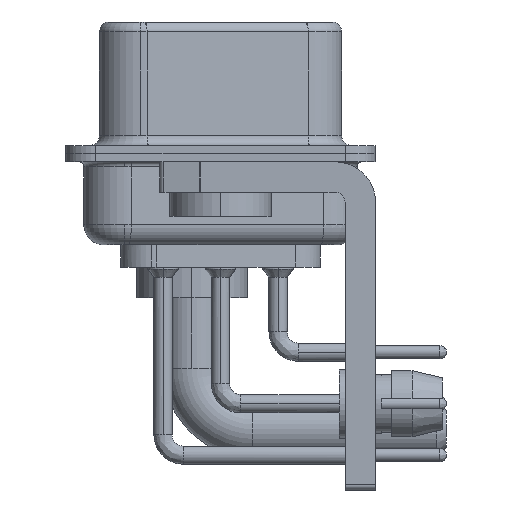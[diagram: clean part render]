
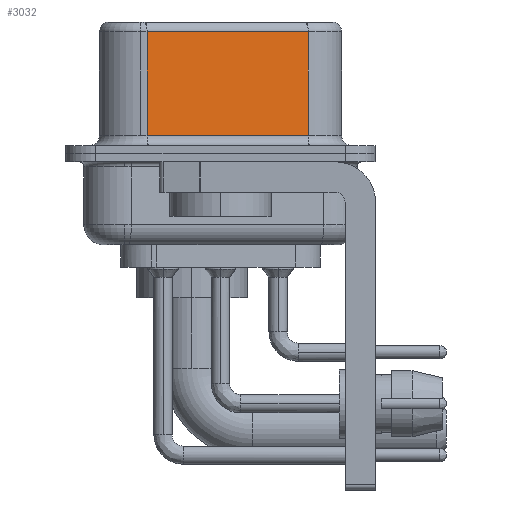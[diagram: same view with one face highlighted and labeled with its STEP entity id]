
A CAD part, left-side view. The second image highlights one B-rep face of the part: STEP entity #3032.
In plain terms, the highlighted planar face has unit normal (-0.985, -0.174, 0).
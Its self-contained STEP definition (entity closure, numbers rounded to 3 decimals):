
#808 = EDGE_CURVE ( 'NONE', #6352, #6250, #20248, .T. ) ;
#848 = VERTEX_POINT ( 'NONE', #11236 ) ;
#2903 = CARTESIAN_POINT ( 'NONE',  ( 5.132, -4.322, 6.02 ) ) ;
#3032 = ADVANCED_FACE ( 'NONE', ( #37084 ), #4297, .F. ) ;
#3439 = VECTOR ( 'NONE', #11633, 1000. ) ;
#4297 = PLANE ( 'NONE',  #15910 ) ;
#6250 = VERTEX_POINT ( 'NONE', #26858 ) ;
#6352 = VERTEX_POINT ( 'NONE', #2903 ) ;
#7738 = ORIENTED_EDGE ( 'NONE', *, *, #22018, .T. ) ;
#8629 = LINE ( 'NONE', #17471, #17528 ) ;
#11236 = CARTESIAN_POINT ( 'NONE',  ( 3.73, 3.628, 0.9 ) ) ;
#11633 = DIRECTION ( 'NONE',  ( -0.174, 0.985, 0. ) ) ;
#12528 = LINE ( 'NONE', #19176, #27349 ) ;
#12939 = DIRECTION ( 'NONE',  ( -0.174, 0.985, 0. ) ) ;
#13773 = EDGE_LOOP ( 'NONE', ( #18597, #20297, #7738, #29267 ) ) ;
#15324 = VERTEX_POINT ( 'NONE', #26922 ) ;
#15433 = VECTOR ( 'NONE', #23337, 1000. ) ;
#15910 = AXIS2_PLACEMENT_3D ( 'NONE', #18819, #22155, #12939 ) ;
#17471 = CARTESIAN_POINT ( 'NONE',  ( 5.132, -4.322, 0.9 ) ) ;
#17528 = VECTOR ( 'NONE', #32004, 1000. ) ;
#18180 = EDGE_CURVE ( 'NONE', #848, #15324, #8629, .T. ) ;
#18597 = ORIENTED_EDGE ( 'NONE', *, *, #21776, .F. ) ;
#18819 = CARTESIAN_POINT ( 'NONE',  ( 5.132, -4.322, 6.52 ) ) ;
#19176 = CARTESIAN_POINT ( 'NONE',  ( 3.73, 3.628, 6.52 ) ) ;
#20248 = LINE ( 'NONE', #38522, #3439 ) ;
#20297 = ORIENTED_EDGE ( 'NONE', *, *, #808, .T. ) ;
#21776 = EDGE_CURVE ( 'NONE', #6352, #15324, #23139, .T. ) ;
#22018 = EDGE_CURVE ( 'NONE', #6250, #848, #12528, .T. ) ;
#22155 = DIRECTION ( 'NONE',  ( 0.985, 0.174, 0. ) ) ;
#23139 = LINE ( 'NONE', #28462, #15433 ) ;
#23337 = DIRECTION ( 'NONE',  ( 0., 0., -1. ) ) ;
#26858 = CARTESIAN_POINT ( 'NONE',  ( 3.73, 3.628, 6.02 ) ) ;
#26922 = CARTESIAN_POINT ( 'NONE',  ( 5.132, -4.322, 0.9 ) ) ;
#27349 = VECTOR ( 'NONE', #36667, 1000. ) ;
#28462 = CARTESIAN_POINT ( 'NONE',  ( 5.132, -4.322, 6.52 ) ) ;
#29267 = ORIENTED_EDGE ( 'NONE', *, *, #18180, .T. ) ;
#32004 = DIRECTION ( 'NONE',  ( 0.174, -0.985, 0. ) ) ;
#36667 = DIRECTION ( 'NONE',  ( 0., 0., -1. ) ) ;
#37084 = FACE_OUTER_BOUND ( 'NONE', #13773, .T. ) ;
#38522 = CARTESIAN_POINT ( 'NONE',  ( 5.132, -4.322, 6.02 ) ) ;
